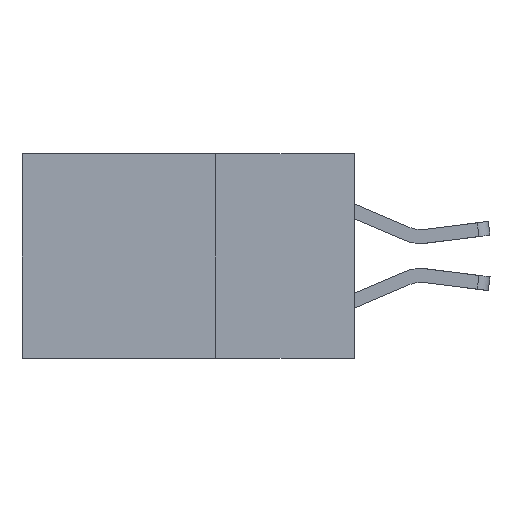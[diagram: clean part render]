
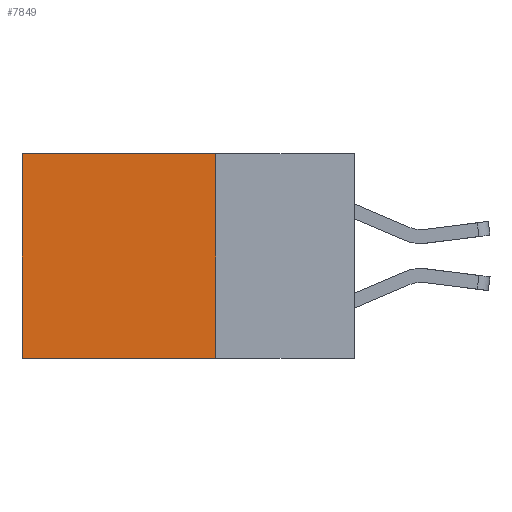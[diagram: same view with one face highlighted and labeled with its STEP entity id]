
A CAD part, left-side view. The second image highlights one B-rep face of the part: STEP entity #7849.
In plain terms, the highlighted planar face has unit normal (-1, 0, 0).
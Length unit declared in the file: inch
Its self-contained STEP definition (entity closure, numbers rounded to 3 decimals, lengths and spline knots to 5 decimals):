
#97 = DIRECTION ( 'NONE',  ( 0., 0., -1. ) ) ;
#110 = DIRECTION ( 'NONE',  ( 1., 0., 0. ) ) ;
#147 = CARTESIAN_POINT ( 'NONE',  ( 0.2615, 0.25, -0.37 ) ) ;
#160 = PLANE ( 'NONE',  #3133 ) ;
#704 = CARTESIAN_POINT ( 'NONE',  ( 0.2615, 0.6, -0.37 ) ) ;
#1521 = DIRECTION ( 'NONE',  ( 0., 1., 0. ) ) ;
#1542 = CARTESIAN_POINT ( 'NONE',  ( 0.2615, 0.25, 0. ) ) ;
#1822 = DIRECTION ( 'NONE',  ( 0., 0., -1. ) ) ;
#1867 = LINE ( 'NONE', #7778, #9182 ) ;
#2121 = EDGE_CURVE ( 'NONE', #3593, #5266, #4341, .T. ) ;
#2124 = LINE ( 'NONE', #1542, #6201 ) ;
#2171 = LINE ( 'NONE', #7053, #6024 ) ;
#2800 = DIRECTION ( 'NONE',  ( 0., 1., 0. ) ) ;
#2885 = CARTESIAN_POINT ( 'NONE',  ( 0.2615, 0.6, 0. ) ) ;
#3133 = AXIS2_PLACEMENT_3D ( 'NONE', #147, #110, #97 ) ;
#3404 = CARTESIAN_POINT ( 'NONE',  ( 0.2615, 0.25, -0.37 ) ) ;
#3593 = VERTEX_POINT ( 'NONE', #6612 ) ;
#4023 = VERTEX_POINT ( 'NONE', #2885 ) ;
#4072 = ORIENTED_EDGE ( 'NONE', *, *, #8160, .F. ) ;
#4341 = LINE ( 'NONE', #3404, #7423 ) ;
#4375 = EDGE_CURVE ( 'NONE', #3593, #4023, #2124, .T. ) ;
#5266 = VERTEX_POINT ( 'NONE', #7355 ) ;
#5620 = EDGE_CURVE ( 'NONE', #4023, #7745, #1867, .T. ) ;
#5769 = ORIENTED_EDGE ( 'NONE', *, *, #5620, .T. ) ;
#5987 = ORIENTED_EDGE ( 'NONE', *, *, #2121, .F. ) ;
#6024 = VECTOR ( 'NONE', #2800, 39.37008 ) ;
#6201 = VECTOR ( 'NONE', #1521, 39.37008 ) ;
#6612 = CARTESIAN_POINT ( 'NONE',  ( 0.2615, 0.25, 0. ) ) ;
#7053 = CARTESIAN_POINT ( 'NONE',  ( 0.2615, 0.25, -0.37 ) ) ;
#7220 = FACE_OUTER_BOUND ( 'NONE', #7455, .T. ) ;
#7355 = CARTESIAN_POINT ( 'NONE',  ( 0.2615, 0.25, -0.37 ) ) ;
#7423 = VECTOR ( 'NONE', #1822, 39.37008 ) ;
#7455 = EDGE_LOOP ( 'NONE', ( #5769, #4072, #5987, #7834 ) ) ;
#7744 = DIRECTION ( 'NONE',  ( 0., 0., -1. ) ) ;
#7745 = VERTEX_POINT ( 'NONE', #704 ) ;
#7778 = CARTESIAN_POINT ( 'NONE',  ( 0.2615, 0.6, -0.37 ) ) ;
#7834 = ORIENTED_EDGE ( 'NONE', *, *, #4375, .T. ) ;
#7849 = ADVANCED_FACE ( 'NONE', ( #7220 ), #160, .F. ) ;
#8160 = EDGE_CURVE ( 'NONE', #5266, #7745, #2171, .T. ) ;
#9182 = VECTOR ( 'NONE', #7744, 39.37008 ) ;
